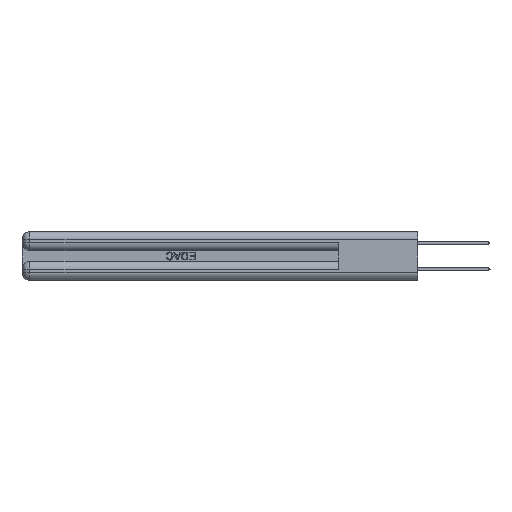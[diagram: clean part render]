
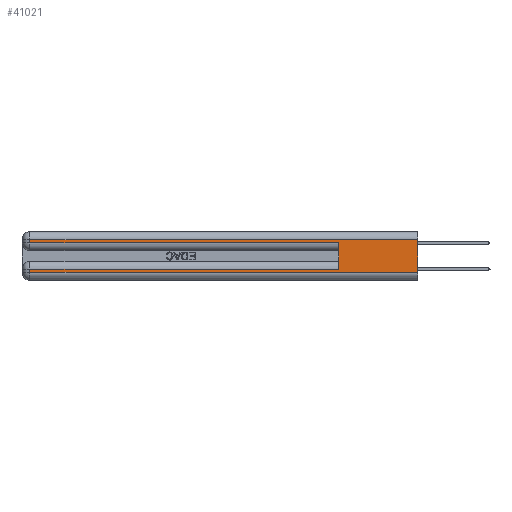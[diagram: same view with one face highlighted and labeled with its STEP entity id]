
A CAD part, left-side view. The second image highlights one B-rep face of the part: STEP entity #41021.
In plain terms, the highlighted planar face has unit normal (-1, 0, 0).
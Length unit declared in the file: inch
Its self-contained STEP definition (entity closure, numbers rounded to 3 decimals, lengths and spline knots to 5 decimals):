
#1365 = CARTESIAN_POINT ( 'NONE',  ( 0., 2.94, 0.06 ) ) ;
#1431 = LINE ( 'NONE', #41773, #27944 ) ;
#1607 = FACE_OUTER_BOUND ( 'NONE', #44260, .T. ) ;
#2128 = CARTESIAN_POINT ( 'NONE',  ( 0., 2.94, 0.37 ) ) ;
#3475 = EDGE_CURVE ( 'NONE', #5871, #43498, #6120, .T. ) ;
#3591 = EDGE_CURVE ( 'NONE', #41665, #8956, #20806, .T. ) ;
#3764 = LINE ( 'NONE', #2128, #32481 ) ;
#4009 = ORIENTED_EDGE ( 'NONE', *, *, #5258, .F. ) ;
#4144 = DIRECTION ( 'NONE',  ( 0., 1., 0. ) ) ;
#4802 = LINE ( 'NONE', #15493, #27894 ) ;
#5258 = EDGE_CURVE ( 'NONE', #19700, #38550, #29085, .T. ) ;
#5390 = DIRECTION ( 'NONE',  ( 1., 0., 0. ) ) ;
#5871 = VERTEX_POINT ( 'NONE', #14016 ) ;
#6120 = LINE ( 'NONE', #9972, #42144 ) ;
#6327 = ORIENTED_EDGE ( 'NONE', *, *, #42397, .T. ) ;
#8956 = VERTEX_POINT ( 'NONE', #10492 ) ;
#9086 = CARTESIAN_POINT ( 'NONE',  ( 0., 0., 0.37 ) ) ;
#9972 = CARTESIAN_POINT ( 'NONE',  ( 0., 0., 0.31 ) ) ;
#10492 = CARTESIAN_POINT ( 'NONE',  ( 0., 0., 0.06 ) ) ;
#12718 = PLANE ( 'NONE',  #42792 ) ;
#13210 = DIRECTION ( 'NONE',  ( 0., -1., 0. ) ) ;
#13274 = EDGE_CURVE ( 'NONE', #19700, #43859, #28095, .T. ) ;
#13599 = DIRECTION ( 'NONE',  ( 0., 1., 0. ) ) ;
#14016 = CARTESIAN_POINT ( 'NONE',  ( 0., 0., 0.31 ) ) ;
#14939 = EDGE_CURVE ( 'NONE', #5871, #8956, #44222, .T. ) ;
#15493 = CARTESIAN_POINT ( 'NONE',  ( 0., 2.94, 0.37 ) ) ;
#15606 = VECTOR ( 'NONE', #19589, 39.37008 ) ;
#15980 = CARTESIAN_POINT ( 'NONE',  ( 0., 0., 0.37 ) ) ;
#16093 = CARTESIAN_POINT ( 'NONE',  ( 0., 0.6, 0.085 ) ) ;
#16336 = DIRECTION ( 'NONE',  ( 0., 0., -1. ) ) ;
#16596 = CARTESIAN_POINT ( 'NONE',  ( 0., 2.94, 0.31 ) ) ;
#18482 = VECTOR ( 'NONE', #32537, 39.37008 ) ;
#18595 = VECTOR ( 'NONE', #4144, 39.37008 ) ;
#19589 = DIRECTION ( 'NONE',  ( 0., 0., -1. ) ) ;
#19700 = VERTEX_POINT ( 'NONE', #16093 ) ;
#20387 = CARTESIAN_POINT ( 'NONE',  ( 0., 2.94, 0.285 ) ) ;
#20806 = LINE ( 'NONE', #35720, #38785 ) ;
#21033 = CARTESIAN_POINT ( 'NONE',  ( 0., 0.6, 0.285 ) ) ;
#22025 = VERTEX_POINT ( 'NONE', #20387 ) ;
#22940 = CARTESIAN_POINT ( 'NONE',  ( 0., 2.94, 0.085 ) ) ;
#25035 = DIRECTION ( 'NONE',  ( 0., -1., 0. ) ) ;
#25937 = ORIENTED_EDGE ( 'NONE', *, *, #3591, .T. ) ;
#26277 = DIRECTION ( 'NONE',  ( 0., 0., -1. ) ) ;
#26535 = EDGE_CURVE ( 'NONE', #43498, #22025, #4802, .T. ) ;
#27894 = VECTOR ( 'NONE', #26277, 39.37008 ) ;
#27944 = VECTOR ( 'NONE', #13210, 39.37008 ) ;
#28095 = LINE ( 'NONE', #32777, #18595 ) ;
#29085 = LINE ( 'NONE', #43237, #18482 ) ;
#32481 = VECTOR ( 'NONE', #41658, 39.37008 ) ;
#32537 = DIRECTION ( 'NONE',  ( 0., 0., 1. ) ) ;
#32777 = CARTESIAN_POINT ( 'NONE',  ( 0., 0., 0.085 ) ) ;
#33170 = ORIENTED_EDGE ( 'NONE', *, *, #26535, .T. ) ;
#35720 = CARTESIAN_POINT ( 'NONE',  ( 0., 0., 0.06 ) ) ;
#38550 = VERTEX_POINT ( 'NONE', #21033 ) ;
#38785 = VECTOR ( 'NONE', #25035, 39.37008 ) ;
#38791 = ORIENTED_EDGE ( 'NONE', *, *, #13274, .T. ) ;
#40181 = ORIENTED_EDGE ( 'NONE', *, *, #14939, .F. ) ;
#41021 = ADVANCED_FACE ( 'NONE', ( #1607 ), #12718, .F. ) ;
#41658 = DIRECTION ( 'NONE',  ( 0., 0., -1. ) ) ;
#41665 = VERTEX_POINT ( 'NONE', #1365 ) ;
#41773 = CARTESIAN_POINT ( 'NONE',  ( 0., 0., 0.285 ) ) ;
#41899 = ORIENTED_EDGE ( 'NONE', *, *, #44043, .T. ) ;
#42144 = VECTOR ( 'NONE', #13599, 39.37008 ) ;
#42397 = EDGE_CURVE ( 'NONE', #43859, #41665, #3764, .T. ) ;
#42792 = AXIS2_PLACEMENT_3D ( 'NONE', #9086, #5390, #16336 ) ;
#43237 = CARTESIAN_POINT ( 'NONE',  ( 0., 0.6, 0.145 ) ) ;
#43498 = VERTEX_POINT ( 'NONE', #16596 ) ;
#43859 = VERTEX_POINT ( 'NONE', #22940 ) ;
#44043 = EDGE_CURVE ( 'NONE', #22025, #38550, #1431, .T. ) ;
#44222 = LINE ( 'NONE', #15980, #15606 ) ;
#44260 = EDGE_LOOP ( 'NONE', ( #40181, #46416, #33170, #41899, #4009, #38791, #6327, #25937 ) ) ;
#46416 = ORIENTED_EDGE ( 'NONE', *, *, #3475, .T. ) ;
